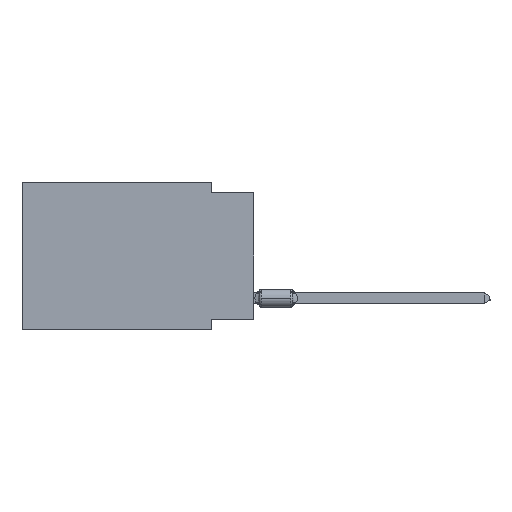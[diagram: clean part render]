
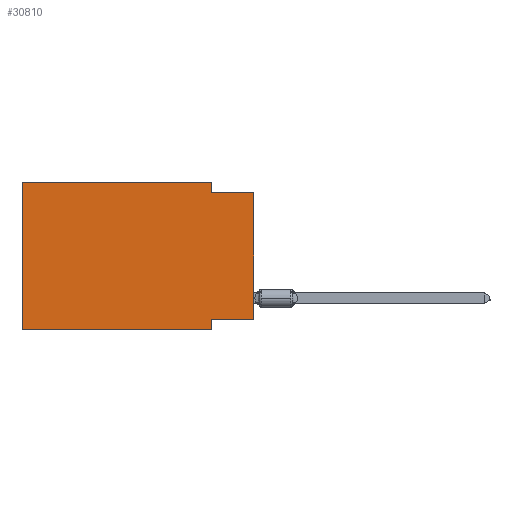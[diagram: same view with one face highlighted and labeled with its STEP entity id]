
A CAD part, left-side view. The second image highlights one B-rep face of the part: STEP entity #30810.
In plain terms, the highlighted planar face has unit normal (-1, 0, 0).
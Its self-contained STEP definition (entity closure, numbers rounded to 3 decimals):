
#207 = ORIENTED_EDGE ( 'NONE', *, *, #19421, .F. ) ;
#303 = CARTESIAN_POINT ( 'NONE',  ( 0., 0., -8.255 ) ) ;
#441 = CARTESIAN_POINT ( 'NONE',  ( 0., 2.54, 0. ) ) ;
#1121 = VERTEX_POINT ( 'NONE', #441 ) ;
#1162 = ORIENTED_EDGE ( 'NONE', *, *, #32750, .F. ) ;
#1184 = PLANE ( 'NONE',  #22911 ) ;
#1461 = ORIENTED_EDGE ( 'NONE', *, *, #24898, .F. ) ;
#1918 = CARTESIAN_POINT ( 'NONE',  ( 0., 0., -0.635 ) ) ;
#3085 = VERTEX_POINT ( 'NONE', #5803 ) ;
#3933 = CARTESIAN_POINT ( 'NONE',  ( 0., 13.97, 0. ) ) ;
#4027 = LINE ( 'NONE', #19491, #17538 ) ;
#4188 = DIRECTION ( 'NONE',  ( 0., 0., -1. ) ) ;
#5769 = DIRECTION ( 'NONE',  ( 0., 0., 1. ) ) ;
#5803 = CARTESIAN_POINT ( 'NONE',  ( 0., 0., -8.255 ) ) ;
#6050 = CARTESIAN_POINT ( 'NONE',  ( 0., 0., -0.635 ) ) ;
#6999 = CARTESIAN_POINT ( 'NONE',  ( 0., 2.54, -8.89 ) ) ;
#8616 = ORIENTED_EDGE ( 'NONE', *, *, #36946, .F. ) ;
#9025 = CARTESIAN_POINT ( 'NONE',  ( 0., 2.54, -0.635 ) ) ;
#10309 = VERTEX_POINT ( 'NONE', #9025 ) ;
#10866 = CARTESIAN_POINT ( 'NONE',  ( 0., 2.54, 0. ) ) ;
#11145 = ORIENTED_EDGE ( 'NONE', *, *, #36219, .F. ) ;
#11594 = EDGE_CURVE ( 'NONE', #21468, #21349, #19465, .T. ) ;
#11990 = ORIENTED_EDGE ( 'NONE', *, *, #20475, .F. ) ;
#12216 = CARTESIAN_POINT ( 'NONE',  ( 0., 13.97, 0. ) ) ;
#12603 = VECTOR ( 'NONE', #37507, 1000. ) ;
#13608 = CARTESIAN_POINT ( 'NONE',  ( 0., 13.97, -8.89 ) ) ;
#13739 = VECTOR ( 'NONE', #14654, 1000. ) ;
#14654 = DIRECTION ( 'NONE',  ( 0., -1., 0. ) ) ;
#16577 = CARTESIAN_POINT ( 'NONE',  ( 0., 13.97, -8.89 ) ) ;
#17538 = VECTOR ( 'NONE', #26353, 1000. ) ;
#18101 = FACE_OUTER_BOUND ( 'NONE', #38624, .T. ) ;
#18583 = ORIENTED_EDGE ( 'NONE', *, *, #30851, .T. ) ;
#19298 = LINE ( 'NONE', #303, #29404 ) ;
#19421 = EDGE_CURVE ( 'NONE', #20624, #21349, #4027, .T. ) ;
#19465 = LINE ( 'NONE', #13608, #40149 ) ;
#19491 = CARTESIAN_POINT ( 'NONE',  ( 0., 2.54, -8.89 ) ) ;
#19867 = DIRECTION ( 'NONE',  ( 0., -1., 0. ) ) ;
#20397 = DIRECTION ( 'NONE',  ( 0., 0., -1. ) ) ;
#20475 = EDGE_CURVE ( 'NONE', #21468, #36718, #21612, .T. ) ;
#20624 = VERTEX_POINT ( 'NONE', #32569 ) ;
#21349 = VERTEX_POINT ( 'NONE', #6999 ) ;
#21468 = VERTEX_POINT ( 'NONE', #16577 ) ;
#21612 = LINE ( 'NONE', #12216, #24271 ) ;
#22719 = VERTEX_POINT ( 'NONE', #6050 ) ;
#22911 = AXIS2_PLACEMENT_3D ( 'NONE', #26633, #36249, #20397 ) ;
#23035 = DIRECTION ( 'NONE',  ( 0., 1., 0. ) ) ;
#23572 = VECTOR ( 'NONE', #34563, 1000. ) ;
#24271 = VECTOR ( 'NONE', #5769, 1000. ) ;
#24364 = ORIENTED_EDGE ( 'NONE', *, *, #11594, .T. ) ;
#24557 = CARTESIAN_POINT ( 'NONE',  ( 0., 0., 0. ) ) ;
#24760 = LINE ( 'NONE', #24557, #23572 ) ;
#24898 = EDGE_CURVE ( 'NONE', #3085, #20624, #19298, .T. ) ;
#26353 = DIRECTION ( 'NONE',  ( 0., 0., -1. ) ) ;
#26495 = LINE ( 'NONE', #10866, #35180 ) ;
#26633 = CARTESIAN_POINT ( 'NONE',  ( 0., 13.97, 0. ) ) ;
#29404 = VECTOR ( 'NONE', #23035, 1000. ) ;
#30300 = LINE ( 'NONE', #1918, #13739 ) ;
#30810 = ADVANCED_FACE ( 'NONE', ( #18101 ), #1184, .F. ) ;
#30851 = EDGE_CURVE ( 'NONE', #3085, #22719, #24760, .T. ) ;
#32569 = CARTESIAN_POINT ( 'NONE',  ( 0., 2.54, -8.255 ) ) ;
#32750 = EDGE_CURVE ( 'NONE', #10309, #22719, #30300, .T. ) ;
#34563 = DIRECTION ( 'NONE',  ( 0., 0., 1. ) ) ;
#35180 = VECTOR ( 'NONE', #4188, 1000. ) ;
#36219 = EDGE_CURVE ( 'NONE', #1121, #10309, #26495, .T. ) ;
#36249 = DIRECTION ( 'NONE',  ( 1., 0., 0. ) ) ;
#36718 = VERTEX_POINT ( 'NONE', #3933 ) ;
#36946 = EDGE_CURVE ( 'NONE', #36718, #1121, #38128, .T. ) ;
#37507 = DIRECTION ( 'NONE',  ( 0., -1., 0. ) ) ;
#38128 = LINE ( 'NONE', #38335, #12603 ) ;
#38335 = CARTESIAN_POINT ( 'NONE',  ( 0., 13.97, 0. ) ) ;
#38624 = EDGE_LOOP ( 'NONE', ( #18583, #1162, #11145, #8616, #11990, #24364, #207, #1461 ) ) ;
#40149 = VECTOR ( 'NONE', #19867, 1000. ) ;
